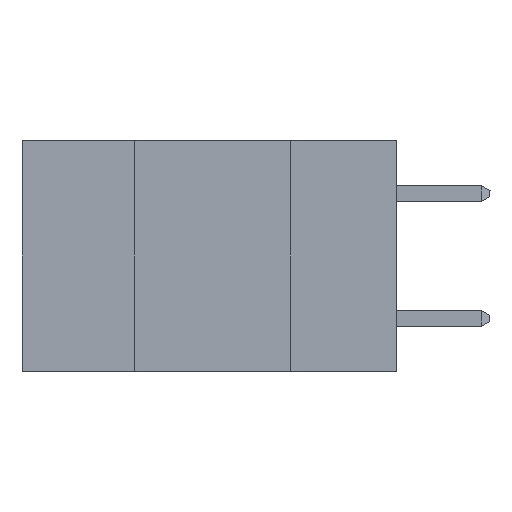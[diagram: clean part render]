
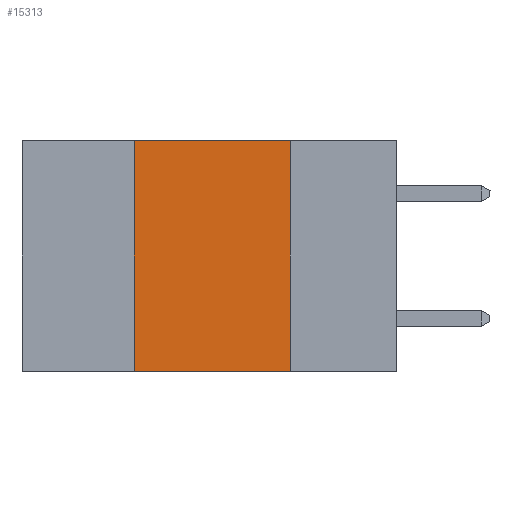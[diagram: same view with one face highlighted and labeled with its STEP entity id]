
A CAD part, left-side view. The second image highlights one B-rep face of the part: STEP entity #15313.
In plain terms, the highlighted planar face has unit normal (-1, 0, 0).
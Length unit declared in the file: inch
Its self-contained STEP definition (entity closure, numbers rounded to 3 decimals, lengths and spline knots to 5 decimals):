
#940 = FACE_OUTER_BOUND ( 'NONE', #9031, .T. ) ;
#1910 = PLANE ( 'NONE',  #16206 ) ;
#2032 = LINE ( 'NONE', #21173, #6893 ) ;
#2072 = CARTESIAN_POINT ( 'NONE',  ( 0., 0.42, 0. ) ) ;
#3451 = VERTEX_POINT ( 'NONE', #14171 ) ;
#4077 = DIRECTION ( 'NONE',  ( 0., 0., -1. ) ) ;
#5432 = LINE ( 'NONE', #21467, #21114 ) ;
#6053 = DIRECTION ( 'NONE',  ( 0., -1., 0. ) ) ;
#6893 = VECTOR ( 'NONE', #25117, 39.37008 ) ;
#7211 = LINE ( 'NONE', #18362, #9152 ) ;
#8442 = EDGE_CURVE ( 'NONE', #17698, #3451, #2032, .T. ) ;
#9031 = EDGE_LOOP ( 'NONE', ( #21118, #18647, #22664, #24462 ) ) ;
#9152 = VECTOR ( 'NONE', #6053, 39.37008 ) ;
#9297 = VERTEX_POINT ( 'NONE', #13634 ) ;
#11363 = EDGE_CURVE ( 'NONE', #9297, #13731, #21355, .T. ) ;
#13634 = CARTESIAN_POINT ( 'NONE',  ( 0., 0.42, -0.37 ) ) ;
#13731 = VERTEX_POINT ( 'NONE', #25260 ) ;
#14017 = CARTESIAN_POINT ( 'NONE',  ( 0., 0.17, 0. ) ) ;
#14171 = CARTESIAN_POINT ( 'NONE',  ( 0., 0.17, -0.37 ) ) ;
#15313 = ADVANCED_FACE ( 'NONE', ( #940 ), #1910, .F. ) ;
#15993 = VECTOR ( 'NONE', #18546, 39.37008 ) ;
#16206 = AXIS2_PLACEMENT_3D ( 'NONE', #22372, #16427, #4077 ) ;
#16427 = DIRECTION ( 'NONE',  ( 1., 0., 0. ) ) ;
#16705 = EDGE_CURVE ( 'NONE', #9297, #3451, #5432, .T. ) ;
#17698 = VERTEX_POINT ( 'NONE', #14017 ) ;
#18362 = CARTESIAN_POINT ( 'NONE',  ( 0., 0.6, 0. ) ) ;
#18546 = DIRECTION ( 'NONE',  ( 0., 0., 1. ) ) ;
#18647 = ORIENTED_EDGE ( 'NONE', *, *, #19698, .F. ) ;
#19698 = EDGE_CURVE ( 'NONE', #13731, #17698, #7211, .T. ) ;
#21114 = VECTOR ( 'NONE', #23452, 39.37008 ) ;
#21118 = ORIENTED_EDGE ( 'NONE', *, *, #8442, .F. ) ;
#21173 = CARTESIAN_POINT ( 'NONE',  ( 0., 0.17, 0. ) ) ;
#21355 = LINE ( 'NONE', #2072, #15993 ) ;
#21467 = CARTESIAN_POINT ( 'NONE',  ( 0., 0.6, -0.37 ) ) ;
#22372 = CARTESIAN_POINT ( 'NONE',  ( 0., 0.6, 0. ) ) ;
#22664 = ORIENTED_EDGE ( 'NONE', *, *, #11363, .F. ) ;
#23452 = DIRECTION ( 'NONE',  ( 0., -1., 0. ) ) ;
#24462 = ORIENTED_EDGE ( 'NONE', *, *, #16705, .T. ) ;
#25117 = DIRECTION ( 'NONE',  ( 0., 0., -1. ) ) ;
#25260 = CARTESIAN_POINT ( 'NONE',  ( 0., 0.42, 0. ) ) ;
